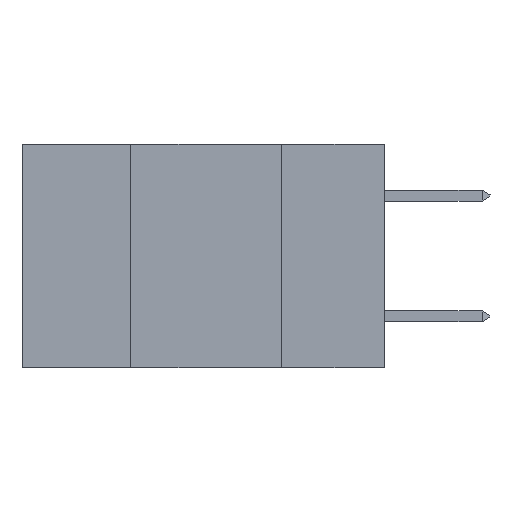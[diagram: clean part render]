
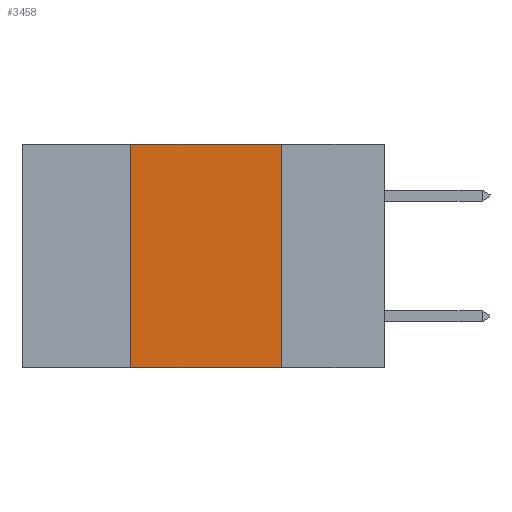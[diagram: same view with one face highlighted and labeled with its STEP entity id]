
A CAD part, left-side view. The second image highlights one B-rep face of the part: STEP entity #3458.
In plain terms, the highlighted planar face has unit normal (-1, 0, 0).
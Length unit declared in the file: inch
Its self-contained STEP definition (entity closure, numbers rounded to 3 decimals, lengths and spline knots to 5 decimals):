
#1048 = VERTEX_POINT ( 'NONE', #3913 ) ;
#1585 = EDGE_CURVE ( 'NONE', #5346, #7008, #11038, .T. ) ;
#2035 = VECTOR ( 'NONE', #11294, 39.37008 ) ;
#3192 = LINE ( 'NONE', #7067, #14975 ) ;
#3329 = AXIS2_PLACEMENT_3D ( 'NONE', #10550, #8214, #9199 ) ;
#3458 = ADVANCED_FACE ( 'NONE', ( #5561 ), #8714, .F. ) ;
#3913 = CARTESIAN_POINT ( 'NONE',  ( 0., 0.17, -0.37 ) ) ;
#4109 = CARTESIAN_POINT ( 'NONE',  ( 0., 0.6, 0. ) ) ;
#4354 = VERTEX_POINT ( 'NONE', #14654 ) ;
#4398 = ORIENTED_EDGE ( 'NONE', *, *, #6692, .F. ) ;
#4962 = VECTOR ( 'NONE', #11666, 39.37008 ) ;
#5140 = EDGE_LOOP ( 'NONE', ( #5732, #14811, #4398, #11106 ) ) ;
#5202 = VECTOR ( 'NONE', #6605, 39.37008 ) ;
#5346 = VERTEX_POINT ( 'NONE', #13662 ) ;
#5561 = FACE_OUTER_BOUND ( 'NONE', #5140, .T. ) ;
#5732 = ORIENTED_EDGE ( 'NONE', *, *, #8275, .F. ) ;
#6605 = DIRECTION ( 'NONE',  ( 0., -1., 0. ) ) ;
#6692 = EDGE_CURVE ( 'NONE', #4354, #5346, #13684, .T. ) ;
#7008 = VERTEX_POINT ( 'NONE', #8113 ) ;
#7067 = CARTESIAN_POINT ( 'NONE',  ( 0., 0.17, 0. ) ) ;
#8113 = CARTESIAN_POINT ( 'NONE',  ( 0., 0.17, 0. ) ) ;
#8214 = DIRECTION ( 'NONE',  ( 1., 0., 0. ) ) ;
#8275 = EDGE_CURVE ( 'NONE', #7008, #1048, #3192, .T. ) ;
#8714 = PLANE ( 'NONE',  #3329 ) ;
#8911 = CARTESIAN_POINT ( 'NONE',  ( 0., 0.6, -0.37 ) ) ;
#9199 = DIRECTION ( 'NONE',  ( 0., 0., -1. ) ) ;
#9838 = CARTESIAN_POINT ( 'NONE',  ( 0., 0.42, 0. ) ) ;
#10550 = CARTESIAN_POINT ( 'NONE',  ( 0., 0.6, 0. ) ) ;
#10590 = DIRECTION ( 'NONE',  ( 0., 0., -1. ) ) ;
#10597 = EDGE_CURVE ( 'NONE', #4354, #1048, #14251, .T. ) ;
#11038 = LINE ( 'NONE', #4109, #2035 ) ;
#11106 = ORIENTED_EDGE ( 'NONE', *, *, #10597, .T. ) ;
#11294 = DIRECTION ( 'NONE',  ( 0., -1., 0. ) ) ;
#11666 = DIRECTION ( 'NONE',  ( 0., 0., 1. ) ) ;
#13662 = CARTESIAN_POINT ( 'NONE',  ( 0., 0.42, 0. ) ) ;
#13684 = LINE ( 'NONE', #9838, #4962 ) ;
#14251 = LINE ( 'NONE', #8911, #5202 ) ;
#14654 = CARTESIAN_POINT ( 'NONE',  ( 0., 0.42, -0.37 ) ) ;
#14811 = ORIENTED_EDGE ( 'NONE', *, *, #1585, .F. ) ;
#14975 = VECTOR ( 'NONE', #10590, 39.37008 ) ;
